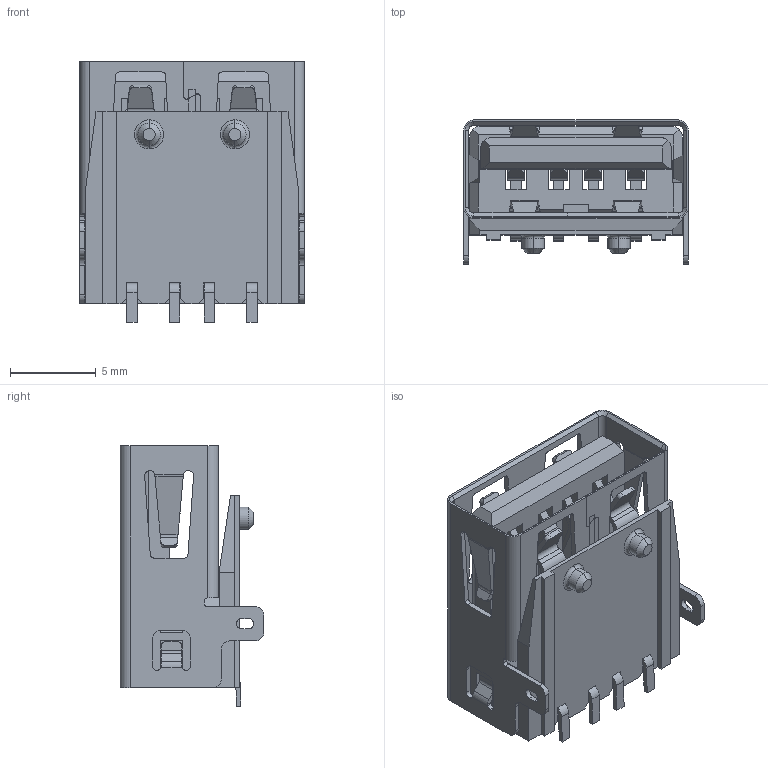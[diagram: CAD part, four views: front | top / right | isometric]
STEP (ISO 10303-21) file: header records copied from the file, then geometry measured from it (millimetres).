
FILE_DESCRIPTION (( 'STEP AP214' ), '1' );
FILE_NAME ('690J104-267-211.STEP', '2021-01-14T13:52:02', ( '' ), ( '' ), 'SwSTEP 2.0', 'SolidWorks 2020', '' );
FILE_SCHEMA (( 'AUTOMOTIVE_DESIGN' ));
Length unit declared in the file: millimetre
Products named in the file (4): Insulator 690J104-X67-21X_Black; 690J104-267-211; Shell 690J104-X67-21X; Contact 690J104-X67-21X
Assembly tree (6 placements, depth 2):
  690J104-267-211
    Insulator 690J104-X67-21X_Black
    Shell 690J104-X67-21X
    Contact 690J104-X67-21X  x4
Bounding box: 13.1 x 8.39 x 15.2 mm (x, y, z)
Volume: 586 mm3; surface area: 2052.3 mm2
Topology: 6 solids, 6 shells, 844 faces, 2317 edges, 1484 vertices
Faces by surface type: plane 540, cylinder 236, bspline 60, cone 8
Entity records: 21577 total; most frequent: CARTESIAN_POINT 5302, ORIENTED_EDGE 3506, DIRECTION 3141, EDGE_CURVE 1753, VECTOR 1319, LINE 1319, VERTEX_POINT 1112, AXIS2_PLACEMENT_3D 911
